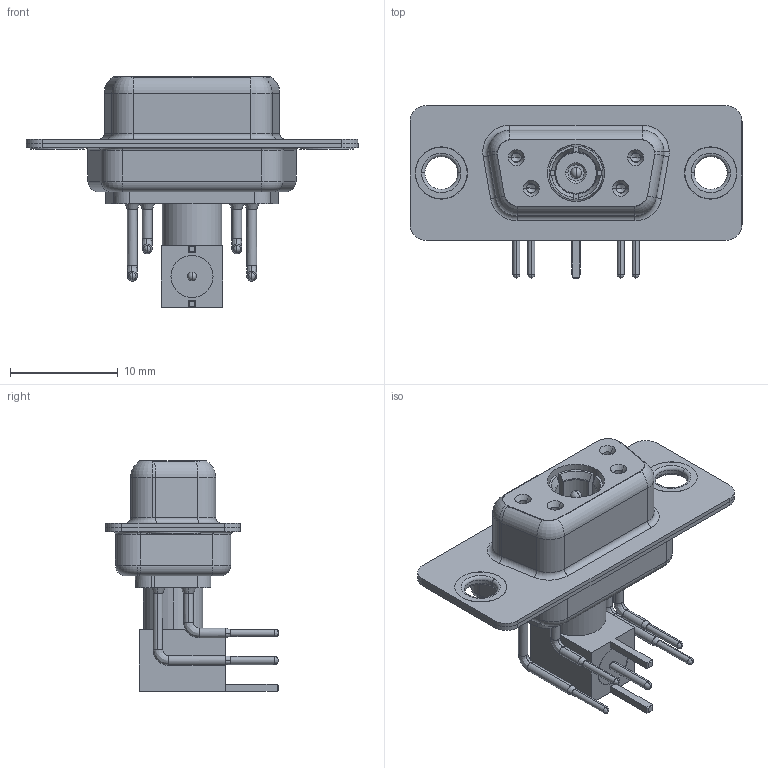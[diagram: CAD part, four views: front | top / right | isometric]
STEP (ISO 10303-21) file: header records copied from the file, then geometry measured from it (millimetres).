
FILE_DESCRIPTION (( 'STEP AP203' ), '1' );
FILE_NAME ('630-5W1-240-7T1.STEP', '2022-05-27T07:55:16', ( '' ), ( '' ), 'SwSTEP 2.0', 'SolidWorks 2020', '' );
FILE_SCHEMA (( 'CONFIG_CONTROL_DESIGN' ));
Length unit declared in the file: millimetre
Products named in the file (14): Insulator Pin_Straight PC Tail; 630Combo Contact Row 2; 630Combo Contact Row 1; 630Combo Shell Rear_09 Contacts; Insulator RA Pin; 630-5W1-240-7T1; 630Combo Shell Front_09 Contacts; Co-Ax Plug_RA PC Tail; RA Back Shell; 630Combo Thru Hole Rivet; Locking Collar; Pin_RA; 630Combo Housing_5W1; Co-Ax Plug Assy_RA
Assembly tree (16 placements, depth 3):
  630-5W1-240-7T1
    630Combo Housing_5W1
    630Combo Shell Front_09 Contacts
    630Combo Shell Rear_09 Contacts
    630Combo Thru Hole Rivet  x2
    Co-Ax Plug Assy_RA
      Co-Ax Plug_RA PC Tail
      Insulator Pin_Straight PC Tail
      Pin_RA
      Locking Collar
      RA Back Shell
      Insulator RA Pin
    630Combo Contact Row 1  x2
    630Combo Contact Row 2  x2
Bounding box: 30.8 x 16 x 21.41 mm (x, y, z)
Volume: 1894.1 mm3; surface area: 4866.4 mm2
Topology: 15 solids, 15 shells, 633 faces, 1544 edges, 962 vertices
Faces by surface type: cylinder 278, plane 194, torus 71, cone 69, bspline 17, sphere 4
Entity records: 17585 total; most frequent: CARTESIAN_POINT 3222, DIRECTION 2909, ORIENTED_EDGE 2540, EDGE_CURVE 1270, AXIS2_PLACEMENT_3D 1182, VERTEX_POINT 802, CIRCLE 638, EDGE_LOOP 606
